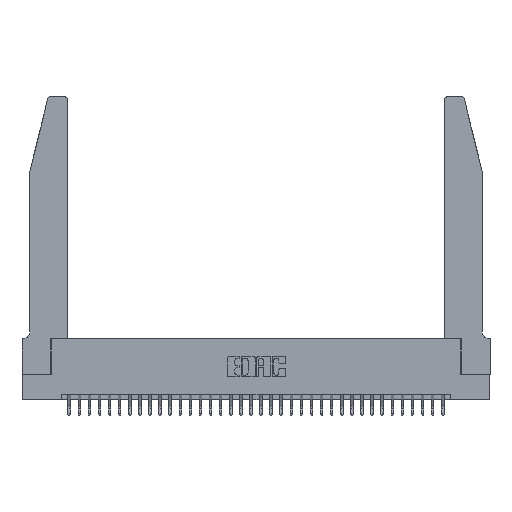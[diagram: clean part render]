
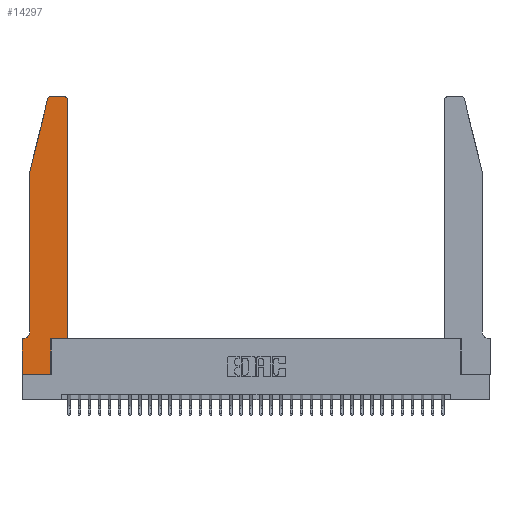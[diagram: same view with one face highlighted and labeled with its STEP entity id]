
A CAD part, top view. The second image highlights one B-rep face of the part: STEP entity #14297.
In plain terms, the highlighted planar face has unit normal (0, 0, 1).
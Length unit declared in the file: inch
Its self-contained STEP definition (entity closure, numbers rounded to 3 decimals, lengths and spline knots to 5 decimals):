
#750 = CARTESIAN_POINT ( 'NONE',  ( 0.0055, 0.42, 0.37 ) ) ;
#1605 = DIRECTION ( 'NONE',  ( 0., 0., 1. ) ) ;
#2254 = DIRECTION ( 'NONE',  ( 0., 1., 0. ) ) ;
#2338 = AXIS2_PLACEMENT_3D ( 'NONE', #750, #33191, #16813 ) ;
#2462 = ORIENTED_EDGE ( 'NONE', *, *, #11653, .T. ) ;
#2652 = CARTESIAN_POINT ( 'NONE',  ( 0., 0., 0.37 ) ) ;
#2822 = CARTESIAN_POINT ( 'NONE',  ( 0.0755, 2., 0.37 ) ) ;
#3059 = DIRECTION ( 'NONE',  ( -0.239, -0.971, 0. ) ) ;
#4555 = VERTEX_POINT ( 'NONE', #24706 ) ;
#4701 = CARTESIAN_POINT ( 'NONE',  ( 0.0755, 2., 0.37 ) ) ;
#5301 = VERTEX_POINT ( 'NONE', #2652 ) ;
#5333 = CARTESIAN_POINT ( 'NONE',  ( 0., 0., 0.37 ) ) ;
#5829 = CARTESIAN_POINT ( 'NONE',  ( 0.0055, 0.35, 0.37 ) ) ;
#5885 = CARTESIAN_POINT ( 'NONE',  ( 0., 0., 0.37 ) ) ;
#6395 = LINE ( 'NONE', #13987, #22170 ) ;
#6481 = DIRECTION ( 'NONE',  ( 1., 0., 0. ) ) ;
#6506 = DIRECTION ( 'NONE',  ( 1., 0., 0. ) ) ;
#7010 = CIRCLE ( 'NONE', #19114, 0.03 ) ;
#7236 = VERTEX_POINT ( 'NONE', #17631 ) ;
#7864 = CARTESIAN_POINT ( 'NONE',  ( 0.4505, 0.35, 0.37 ) ) ;
#8047 = ORIENTED_EDGE ( 'NONE', *, *, #10652, .T. ) ;
#8915 = CARTESIAN_POINT ( 'NONE',  ( 0., 0.35, 0.37 ) ) ;
#10537 = DIRECTION ( 'NONE',  ( 1., 0., 0. ) ) ;
#10652 = EDGE_CURVE ( 'NONE', #21821, #30896, #26552, .T. ) ;
#10752 = VECTOR ( 'NONE', #2254, 39.37008 ) ;
#10992 = DIRECTION ( 'NONE',  ( 0., -1., 0. ) ) ;
#11387 = EDGE_CURVE ( 'NONE', #4555, #22364, #23946, .T. ) ;
#11461 = FACE_OUTER_BOUND ( 'NONE', #16951, .T. ) ;
#11491 = CARTESIAN_POINT ( 'NONE',  ( 0., 0.35, 0.37 ) ) ;
#11625 = CARTESIAN_POINT ( 'NONE',  ( 0.2865, 0., 0.37 ) ) ;
#11653 = EDGE_CURVE ( 'NONE', #30896, #13012, #18361, .T. ) ;
#12201 = DIRECTION ( 'NONE',  ( 0., 1., 0. ) ) ;
#12579 = CARTESIAN_POINT ( 'NONE',  ( 0.284, 2.75, 0.37 ) ) ;
#12930 = CARTESIAN_POINT ( 'NONE',  ( 0.0755, 0.35, 0.37 ) ) ;
#12962 = AXIS2_PLACEMENT_3D ( 'NONE', #23126, #1605, #20634 ) ;
#13012 = VERTEX_POINT ( 'NONE', #7864 ) ;
#13616 = AXIS2_PLACEMENT_3D ( 'NONE', #11491, #14145, #16872 ) ;
#13987 = CARTESIAN_POINT ( 'NONE',  ( 0.0755, 2., 0.37 ) ) ;
#14145 = DIRECTION ( 'NONE',  ( 0., 0., 1. ) ) ;
#14154 = ORIENTED_EDGE ( 'NONE', *, *, #16483, .T. ) ;
#14297 = ADVANCED_FACE ( 'NONE', ( #11461 ), #30466, .T. ) ;
#14379 = VERTEX_POINT ( 'NONE', #5829 ) ;
#14863 = CARTESIAN_POINT ( 'NONE',  ( 0.2605, 2.75, 0.37 ) ) ;
#14983 = LINE ( 'NONE', #2822, #32537 ) ;
#15060 = CARTESIAN_POINT ( 'NONE',  ( 0.2865, 0.35, 0.37 ) ) ;
#15083 = EDGE_CURVE ( 'NONE', #7236, #16636, #6395, .T. ) ;
#16483 = EDGE_CURVE ( 'NONE', #29348, #4555, #23342, .T. ) ;
#16636 = VERTEX_POINT ( 'NONE', #4701 ) ;
#16813 = DIRECTION ( 'NONE',  ( -1., 0., 0. ) ) ;
#16872 = DIRECTION ( 'NONE',  ( 1., 0., 0. ) ) ;
#16951 = EDGE_LOOP ( 'NONE', ( #31894, #30340, #26928, #23163, #26349, #34514, #32097, #19877, #8047, #2462, #28383, #14154 ) ) ;
#17431 = VERTEX_POINT ( 'NONE', #8915 ) ;
#17631 = CARTESIAN_POINT ( 'NONE',  ( 0.25487, 2.72718, 0.37 ) ) ;
#18361 = LINE ( 'NONE', #33791, #30740 ) ;
#18685 = EDGE_CURVE ( 'NONE', #17431, #5301, #21916, .T. ) ;
#19114 = AXIS2_PLACEMENT_3D ( 'NONE', #22793, #25778, #6506 ) ;
#19256 = VECTOR ( 'NONE', #12201, 39.37008 ) ;
#19877 = ORIENTED_EDGE ( 'NONE', *, *, #29044, .T. ) ;
#20634 = DIRECTION ( 'NONE',  ( 1., 0., 0. ) ) ;
#21077 = EDGE_CURVE ( 'NONE', #22031, #14379, #29166, .T. ) ;
#21216 = CARTESIAN_POINT ( 'NONE',  ( 0.0755, 0.42, 0.37 ) ) ;
#21821 = VERTEX_POINT ( 'NONE', #11625 ) ;
#21916 = LINE ( 'NONE', #5885, #26191 ) ;
#21950 = CARTESIAN_POINT ( 'NONE',  ( 0.4505, 2.72, 0.37 ) ) ;
#22031 = VERTEX_POINT ( 'NONE', #21216 ) ;
#22170 = VECTOR ( 'NONE', #3059, 39.37008 ) ;
#22268 = LINE ( 'NONE', #32183, #10752 ) ;
#22364 = VERTEX_POINT ( 'NONE', #12579 ) ;
#22690 = EDGE_CURVE ( 'NONE', #16636, #22031, #14983, .T. ) ;
#22793 = CARTESIAN_POINT ( 'NONE',  ( 0.284, 2.72, 0.37 ) ) ;
#23126 = CARTESIAN_POINT ( 'NONE',  ( 0.4205, 2.72, 0.37 ) ) ;
#23163 = ORIENTED_EDGE ( 'NONE', *, *, #22690, .T. ) ;
#23342 = CIRCLE ( 'NONE', #12962, 0.03 ) ;
#23946 = LINE ( 'NONE', #14863, #34687 ) ;
#24706 = CARTESIAN_POINT ( 'NONE',  ( 0.4205, 2.75, 0.37 ) ) ;
#24919 = DIRECTION ( 'NONE',  ( 0., -1., 0. ) ) ;
#25778 = DIRECTION ( 'NONE',  ( 0., 0., 1. ) ) ;
#26068 = EDGE_CURVE ( 'NONE', #14379, #17431, #33998, .T. ) ;
#26086 = DIRECTION ( 'NONE',  ( -1., 0., 0. ) ) ;
#26191 = VECTOR ( 'NONE', #24919, 39.37008 ) ;
#26349 = ORIENTED_EDGE ( 'NONE', *, *, #21077, .T. ) ;
#26552 = LINE ( 'NONE', #15060, #19256 ) ;
#26708 = VECTOR ( 'NONE', #29486, 39.37008 ) ;
#26928 = ORIENTED_EDGE ( 'NONE', *, *, #15083, .T. ) ;
#28263 = CARTESIAN_POINT ( 'NONE',  ( 0.2865, 0.35, 0.37 ) ) ;
#28341 = LINE ( 'NONE', #5333, #28775 ) ;
#28383 = ORIENTED_EDGE ( 'NONE', *, *, #30474, .T. ) ;
#28775 = VECTOR ( 'NONE', #10537, 39.37008 ) ;
#29044 = EDGE_CURVE ( 'NONE', #5301, #21821, #28341, .T. ) ;
#29166 = CIRCLE ( 'NONE', #2338, 0.07 ) ;
#29348 = VERTEX_POINT ( 'NONE', #21950 ) ;
#29486 = DIRECTION ( 'NONE',  ( -1., 0., 0. ) ) ;
#30340 = ORIENTED_EDGE ( 'NONE', *, *, #35092, .T. ) ;
#30466 = PLANE ( 'NONE',  #13616 ) ;
#30474 = EDGE_CURVE ( 'NONE', #13012, #29348, #22268, .T. ) ;
#30740 = VECTOR ( 'NONE', #6481, 39.37008 ) ;
#30896 = VERTEX_POINT ( 'NONE', #28263 ) ;
#31894 = ORIENTED_EDGE ( 'NONE', *, *, #11387, .T. ) ;
#32097 = ORIENTED_EDGE ( 'NONE', *, *, #18685, .T. ) ;
#32183 = CARTESIAN_POINT ( 'NONE',  ( 0.4505, 0.35, 0.37 ) ) ;
#32537 = VECTOR ( 'NONE', #10992, 39.37008 ) ;
#33191 = DIRECTION ( 'NONE',  ( 0., 0., -1. ) ) ;
#33791 = CARTESIAN_POINT ( 'NONE',  ( 0.4505, 0.35, 0.37 ) ) ;
#33998 = LINE ( 'NONE', #12930, #26708 ) ;
#34514 = ORIENTED_EDGE ( 'NONE', *, *, #26068, .T. ) ;
#34687 = VECTOR ( 'NONE', #26086, 39.37008 ) ;
#35092 = EDGE_CURVE ( 'NONE', #22364, #7236, #7010, .T. ) ;
